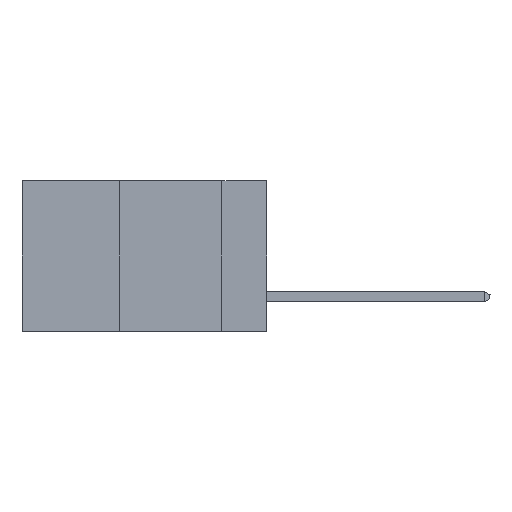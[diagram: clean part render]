
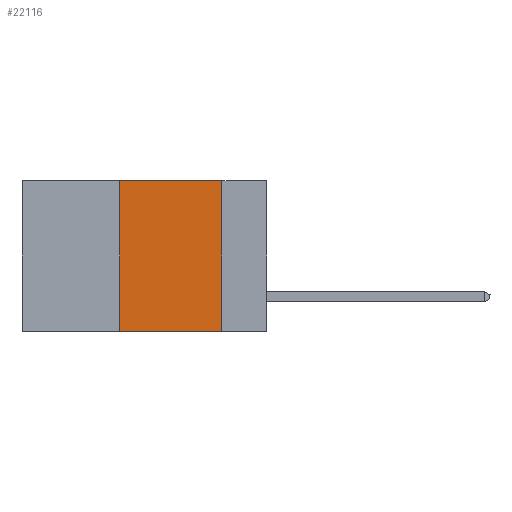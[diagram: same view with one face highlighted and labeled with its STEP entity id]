
A CAD part, left-side view. The second image highlights one B-rep face of the part: STEP entity #22116.
In plain terms, the highlighted planar face has unit normal (-1, 0, 0).
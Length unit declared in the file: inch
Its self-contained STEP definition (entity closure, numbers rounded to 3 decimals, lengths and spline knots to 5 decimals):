
#607 = LINE ( 'NONE', #24910, #15574 ) ;
#968 = VECTOR ( 'NONE', #23025, 39.37008 ) ;
#1447 = DIRECTION ( 'NONE',  ( 1., 0., 0. ) ) ;
#1911 = VERTEX_POINT ( 'NONE', #17335 ) ;
#3243 = EDGE_CURVE ( 'NONE', #1911, #26760, #29434, .T. ) ;
#3273 = DIRECTION ( 'NONE',  ( 0., 0., -1. ) ) ;
#3584 = DIRECTION ( 'NONE',  ( 0., 0., -1. ) ) ;
#3702 = FACE_OUTER_BOUND ( 'NONE', #18721, .T. ) ;
#6043 = CARTESIAN_POINT ( 'NONE',  ( 0., 0.11, -0.37 ) ) ;
#7740 = VERTEX_POINT ( 'NONE', #27264 ) ;
#11397 = ORIENTED_EDGE ( 'NONE', *, *, #21848, .T. ) ;
#11931 = LINE ( 'NONE', #15451, #19190 ) ;
#14416 = ORIENTED_EDGE ( 'NONE', *, *, #3243, .F. ) ;
#14794 = LINE ( 'NONE', #30112, #968 ) ;
#15451 = CARTESIAN_POINT ( 'NONE',  ( 0., 0.36, 0. ) ) ;
#15574 = VECTOR ( 'NONE', #22865, 39.37008 ) ;
#15843 = CARTESIAN_POINT ( 'NONE',  ( 0., 0.11, 0. ) ) ;
#16788 = VECTOR ( 'NONE', #3273, 39.37008 ) ;
#17335 = CARTESIAN_POINT ( 'NONE',  ( 0., 0.11, 0. ) ) ;
#17628 = EDGE_CURVE ( 'NONE', #7740, #19358, #11931, .T. ) ;
#18721 = EDGE_LOOP ( 'NONE', ( #14416, #19079, #19075, #11397 ) ) ;
#19075 = ORIENTED_EDGE ( 'NONE', *, *, #17628, .F. ) ;
#19079 = ORIENTED_EDGE ( 'NONE', *, *, #30555, .F. ) ;
#19190 = VECTOR ( 'NONE', #22630, 39.37008 ) ;
#19358 = VERTEX_POINT ( 'NONE', #29908 ) ;
#20302 = AXIS2_PLACEMENT_3D ( 'NONE', #20847, #1447, #3584 ) ;
#20847 = CARTESIAN_POINT ( 'NONE',  ( 0., 0.6, 0. ) ) ;
#21848 = EDGE_CURVE ( 'NONE', #7740, #26760, #607, .T. ) ;
#22116 = ADVANCED_FACE ( 'NONE', ( #3702 ), #22968, .F. ) ;
#22630 = DIRECTION ( 'NONE',  ( 0., 0., 1. ) ) ;
#22865 = DIRECTION ( 'NONE',  ( 0., -1., 0. ) ) ;
#22968 = PLANE ( 'NONE',  #20302 ) ;
#23025 = DIRECTION ( 'NONE',  ( 0., -1., 0. ) ) ;
#24910 = CARTESIAN_POINT ( 'NONE',  ( 0., 0.6, -0.37 ) ) ;
#26760 = VERTEX_POINT ( 'NONE', #6043 ) ;
#27264 = CARTESIAN_POINT ( 'NONE',  ( 0., 0.36, -0.37 ) ) ;
#29434 = LINE ( 'NONE', #15843, #16788 ) ;
#29908 = CARTESIAN_POINT ( 'NONE',  ( 0., 0.36, 0. ) ) ;
#30112 = CARTESIAN_POINT ( 'NONE',  ( 0., 0.6, 0. ) ) ;
#30555 = EDGE_CURVE ( 'NONE', #19358, #1911, #14794, .T. ) ;
